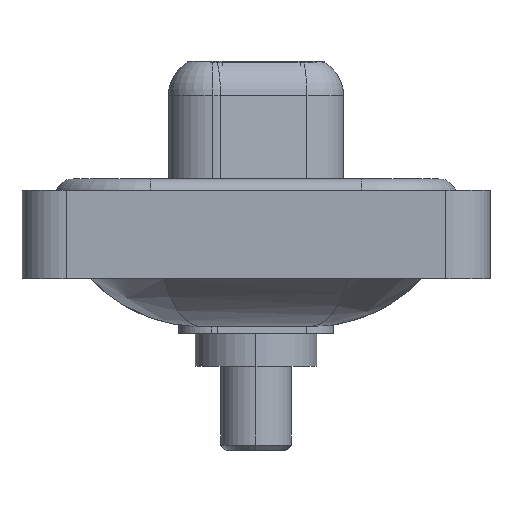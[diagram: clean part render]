
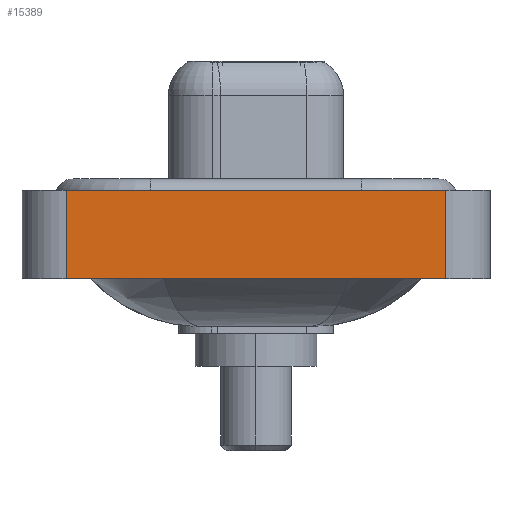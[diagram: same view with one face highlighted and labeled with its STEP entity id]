
A CAD part, left-side view. The second image highlights one B-rep face of the part: STEP entity #15389.
In plain terms, the highlighted planar face has unit normal (-1, 0, 0).
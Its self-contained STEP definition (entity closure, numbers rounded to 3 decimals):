
#885 = CARTESIAN_POINT ( 'NONE',  ( -7.3, 8.55, 0.4 ) ) ;
#922 = AXIS2_PLACEMENT_3D ( 'NONE', #4062, #14680, #5301 ) ;
#1299 = CARTESIAN_POINT ( 'NONE',  ( -7.3, -8.55, 0.4 ) ) ;
#2451 = DIRECTION ( 'NONE',  ( 0., -1., 0. ) ) ;
#2823 = DIRECTION ( 'NONE',  ( 0., 0., 1. ) ) ;
#3387 = CARTESIAN_POINT ( 'NONE',  ( -7.3, -8.55, 0.4 ) ) ;
#3875 = LINE ( 'NONE', #1299, #12532 ) ;
#4001 = LINE ( 'NONE', #9381, #8233 ) ;
#4062 = CARTESIAN_POINT ( 'NONE',  ( -7.3, -8.55, -3.6 ) ) ;
#4942 = VECTOR ( 'NONE', #12834, 1000. ) ;
#5301 = DIRECTION ( 'NONE',  ( 0., 0., 1. ) ) ;
#5388 = LINE ( 'NONE', #9459, #9349 ) ;
#5648 = CARTESIAN_POINT ( 'NONE',  ( -7.3, -8.55, -3.6 ) ) ;
#5933 = DIRECTION ( 'NONE',  ( 0., 0., 1. ) ) ;
#6163 = CARTESIAN_POINT ( 'NONE',  ( -7.3, 8.55, -3.6 ) ) ;
#6755 = EDGE_CURVE ( 'NONE', #17032, #11689, #5388, .T. ) ;
#7427 = LINE ( 'NONE', #11593, #4942 ) ;
#7673 = EDGE_CURVE ( 'NONE', #16863, #15951, #4001, .T. ) ;
#7790 = ORIENTED_EDGE ( 'NONE', *, *, #15770, .F. ) ;
#8233 = VECTOR ( 'NONE', #5933, 1000. ) ;
#9349 = VECTOR ( 'NONE', #2823, 1000. ) ;
#9381 = CARTESIAN_POINT ( 'NONE',  ( -7.3, -8.55, -3.6 ) ) ;
#9459 = CARTESIAN_POINT ( 'NONE',  ( -7.3, 8.55, -3.6 ) ) ;
#9535 = FACE_OUTER_BOUND ( 'NONE', #13576, .T. ) ;
#10433 = EDGE_CURVE ( 'NONE', #17032, #16863, #7427, .T. ) ;
#11593 = CARTESIAN_POINT ( 'NONE',  ( -7.3, -8.55, -3.6 ) ) ;
#11689 = VERTEX_POINT ( 'NONE', #885 ) ;
#12113 = PLANE ( 'NONE',  #922 ) ;
#12532 = VECTOR ( 'NONE', #2451, 1000. ) ;
#12834 = DIRECTION ( 'NONE',  ( 0., -1., 0. ) ) ;
#13576 = EDGE_LOOP ( 'NONE', ( #14030, #7790, #13773, #14435 ) ) ;
#13773 = ORIENTED_EDGE ( 'NONE', *, *, #6755, .F. ) ;
#14030 = ORIENTED_EDGE ( 'NONE', *, *, #7673, .T. ) ;
#14435 = ORIENTED_EDGE ( 'NONE', *, *, #10433, .T. ) ;
#14680 = DIRECTION ( 'NONE',  ( -1., 0., 0. ) ) ;
#15389 = ADVANCED_FACE ( 'NONE', ( #9535 ), #12113, .T. ) ;
#15770 = EDGE_CURVE ( 'NONE', #11689, #15951, #3875, .T. ) ;
#15951 = VERTEX_POINT ( 'NONE', #3387 ) ;
#16863 = VERTEX_POINT ( 'NONE', #5648 ) ;
#17032 = VERTEX_POINT ( 'NONE', #6163 ) ;
